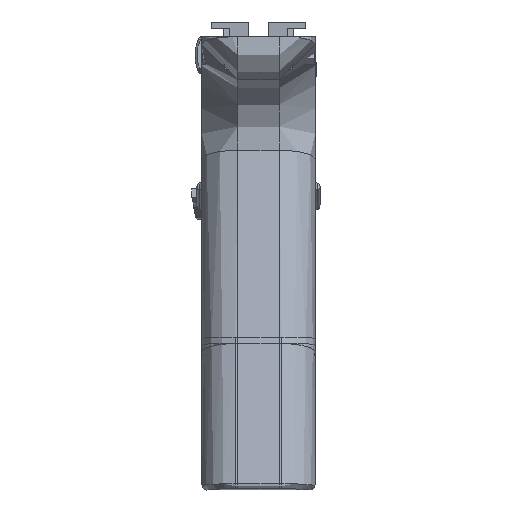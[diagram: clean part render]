
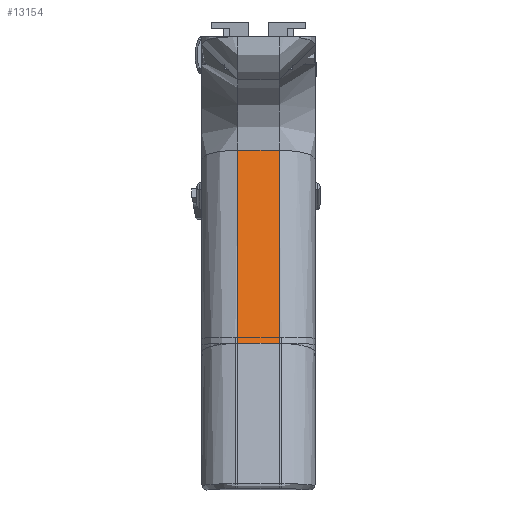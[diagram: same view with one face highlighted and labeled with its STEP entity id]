
A CAD part, front view. The second image highlights one B-rep face of the part: STEP entity #13154.
In plain terms, the highlighted face is planar.
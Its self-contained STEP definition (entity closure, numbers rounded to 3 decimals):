
#1028=PLANE('',#14355);
#1638=FACE_OUTER_BOUND('',#2396,.T.);
#2396=EDGE_LOOP('',(#11389,#11390,#11391,#11392));
#3394=LINE('',#23263,#4564);
#3551=LINE('',#24118,#4721);
#3552=LINE('',#24121,#4722);
#3553=LINE('',#24122,#4723);
#4564=VECTOR('',#16951,10.);
#4721=VECTOR('',#17356,10.);
#4722=VECTOR('',#17359,10.);
#4723=VECTOR('',#17360,10.);
#6155=VERTEX_POINT('',#23259);
#6156=VERTEX_POINT('',#23261);
#6297=VERTEX_POINT('',#24096);
#6300=VERTEX_POINT('',#24120);
#7848=EDGE_CURVE('',#6155,#6156,#3394,.T.);
#8075=EDGE_CURVE('',#6155,#6297,#3551,.T.);
#8076=EDGE_CURVE('',#6300,#6156,#3552,.T.);
#8077=EDGE_CURVE('',#6297,#6300,#3553,.T.);
#11389=ORIENTED_EDGE('',*,*,#8076,.F.);
#11390=ORIENTED_EDGE('',*,*,#8077,.F.);
#11391=ORIENTED_EDGE('',*,*,#8075,.F.);
#11392=ORIENTED_EDGE('',*,*,#7848,.T.);
#13154=ADVANCED_FACE('',(#1638),#1028,.T.);
#14355=AXIS2_PLACEMENT_3D('',#24119,#17357,#17358);
#16951=DIRECTION('',(0.,-0.249,0.969));
#17356=DIRECTION('',(-1.,0.,0.));
#17357=DIRECTION('center_axis',(0.,-0.969,
-0.249));
#17358=DIRECTION('ref_axis',(0.,-0.249,0.969));
#17359=DIRECTION('',(1.,0.,0.));
#17360=DIRECTION('',(0.,-0.249,0.969));
#23259=CARTESIAN_POINT('',(13.45,-71.634,19.877));
#23261=CARTESIAN_POINT('',(13.45,-83.628,66.536));
#23263=CARTESIAN_POINT('',(13.45,-83.554,66.245));
#24096=CARTESIAN_POINT('',(3.45,-71.634,19.877));
#24118=CARTESIAN_POINT('',(22.175,-71.634,19.877));
#24119=CARTESIAN_POINT('Origin',(22.175,-71.634,19.877));
#24120=CARTESIAN_POINT('',(3.45,-83.628,66.536));
#24121=CARTESIAN_POINT('',(22.175,-83.628,66.536));
#24122=CARTESIAN_POINT('',(3.45,-83.554,66.245));
